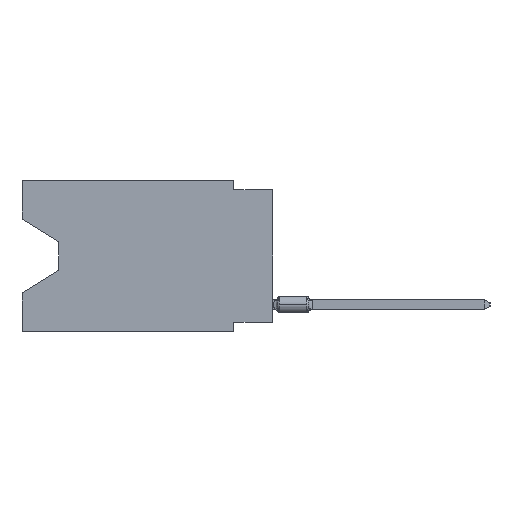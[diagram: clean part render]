
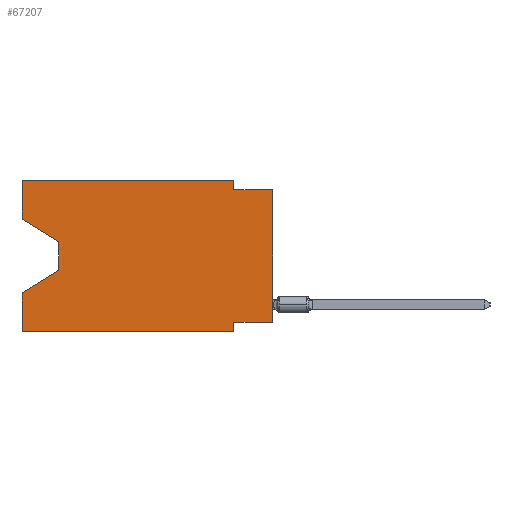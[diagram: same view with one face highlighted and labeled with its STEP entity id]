
A CAD part, left-side view. The second image highlights one B-rep face of the part: STEP entity #67207.
In plain terms, the highlighted planar face has unit normal (-1, 0, 0).
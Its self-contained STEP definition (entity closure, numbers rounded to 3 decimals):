
#865 = VECTOR ( 'NONE', #69409, 1000. ) ;
#2156 = VECTOR ( 'NONE', #59190, 1000. ) ;
#2720 = CARTESIAN_POINT ( 'NONE',  ( 0., 2.54, 0. ) ) ;
#2773 = VECTOR ( 'NONE', #17506, 1000. ) ;
#2806 = CARTESIAN_POINT ( 'NONE',  ( 0., 16.383, -7.36 ) ) ;
#4636 = DIRECTION ( 'NONE',  ( 0., 0.855, -0.519 ) ) ;
#7110 = ORIENTED_EDGE ( 'NONE', *, *, #70631, .F. ) ;
#7750 = VECTOR ( 'NONE', #42938, 1000. ) ;
#7987 = EDGE_CURVE ( 'NONE', #22921, #85334, #28754, .T. ) ;
#11176 = VECTOR ( 'NONE', #67399, 1000. ) ;
#14321 = ORIENTED_EDGE ( 'NONE', *, *, #21573, .F. ) ;
#15529 = EDGE_CURVE ( 'NONE', #75720, #67222, #23640, .T. ) ;
#15747 = CARTESIAN_POINT ( 'NONE',  ( 0., 13.97, -4.013 ) ) ;
#16799 = ORIENTED_EDGE ( 'NONE', *, *, #28957, .F. ) ;
#17506 = DIRECTION ( 'NONE',  ( 0., -1., 0. ) ) ;
#19652 = ORIENTED_EDGE ( 'NONE', *, *, #63104, .T. ) ;
#21573 = EDGE_CURVE ( 'NONE', #85607, #34274, #83770, .T. ) ;
#22626 = CARTESIAN_POINT ( 'NONE',  ( 0., 0., -9.271 ) ) ;
#22858 = VECTOR ( 'NONE', #66157, 1000. ) ;
#22921 = VERTEX_POINT ( 'NONE', #47606 ) ;
#23640 = LINE ( 'NONE', #15747, #7750 ) ;
#25227 = VERTEX_POINT ( 'NONE', #72711 ) ;
#25934 = CARTESIAN_POINT ( 'NONE',  ( 0., 2.54, -0.635 ) ) ;
#26866 = CARTESIAN_POINT ( 'NONE',  ( 0., 16.383, 0. ) ) ;
#27895 = VERTEX_POINT ( 'NONE', #2806 ) ;
#27979 = CARTESIAN_POINT ( 'NONE',  ( 0., 13.97, -4.013 ) ) ;
#28754 = LINE ( 'NONE', #55521, #61513 ) ;
#28957 = EDGE_CURVE ( 'NONE', #41726, #27895, #59170, .T. ) ;
#29472 = LINE ( 'NONE', #30329, #865 ) ;
#29495 = VERTEX_POINT ( 'NONE', #2720 ) ;
#30114 = ORIENTED_EDGE ( 'NONE', *, *, #72258, .F. ) ;
#30329 = CARTESIAN_POINT ( 'NONE',  ( 0., 16.383, -9.906 ) ) ;
#30726 = LINE ( 'NONE', #56609, #71638 ) ;
#30903 = ORIENTED_EDGE ( 'NONE', *, *, #15529, .T. ) ;
#31902 = LINE ( 'NONE', #85434, #78653 ) ;
#31994 = CARTESIAN_POINT ( 'NONE',  ( 0., 16.383, -2.546 ) ) ;
#34274 = VERTEX_POINT ( 'NONE', #86772 ) ;
#34283 = EDGE_CURVE ( 'NONE', #54685, #22921, #37753, .T. ) ;
#34741 = AXIS2_PLACEMENT_3D ( 'NONE', #49999, #68485, #36417 ) ;
#35579 = EDGE_LOOP ( 'NONE', ( #43740, #30903, #40890, #16799, #19652, #63907, #70635, #58955, #14321, #30114, #7110, #37715 ) ) ;
#35743 = LINE ( 'NONE', #40631, #11176 ) ;
#36405 = CARTESIAN_POINT ( 'NONE',  ( 0., 0., -0.635 ) ) ;
#36417 = DIRECTION ( 'NONE',  ( 0., 0., -1. ) ) ;
#37715 = ORIENTED_EDGE ( 'NONE', *, *, #39222, .F. ) ;
#37753 = LINE ( 'NONE', #71112, #22858 ) ;
#39222 = EDGE_CURVE ( 'NONE', #72754, #25227, #60225, .T. ) ;
#40631 = CARTESIAN_POINT ( 'NONE',  ( 0., 16.383, 0. ) ) ;
#40890 = ORIENTED_EDGE ( 'NONE', *, *, #60741, .T. ) ;
#41726 = VERTEX_POINT ( 'NONE', #45066 ) ;
#42938 = DIRECTION ( 'NONE',  ( 0., 0., -1. ) ) ;
#43740 = ORIENTED_EDGE ( 'NONE', *, *, #56161, .T. ) ;
#44556 = LINE ( 'NONE', #64737, #75453 ) ;
#45066 = CARTESIAN_POINT ( 'NONE',  ( 0., 16.383, -9.906 ) ) ;
#47606 = CARTESIAN_POINT ( 'NONE',  ( 0., 2.54, -9.271 ) ) ;
#49999 = CARTESIAN_POINT ( 'NONE',  ( 0., 16.383, 0. ) ) ;
#54685 = VERTEX_POINT ( 'NONE', #22626 ) ;
#55287 = FACE_OUTER_BOUND ( 'NONE', #35579, .T. ) ;
#55521 = CARTESIAN_POINT ( 'NONE',  ( 0., 2.54, -9.906 ) ) ;
#56161 = EDGE_CURVE ( 'NONE', #72754, #75720, #58296, .T. ) ;
#56609 = CARTESIAN_POINT ( 'NONE',  ( 0., 0., 0. ) ) ;
#58204 = DIRECTION ( 'NONE',  ( 0., 0., -1. ) ) ;
#58296 = LINE ( 'NONE', #31994, #2156 ) ;
#58955 = ORIENTED_EDGE ( 'NONE', *, *, #78268, .T. ) ;
#59170 = LINE ( 'NONE', #86356, #81744 ) ;
#59190 = DIRECTION ( 'NONE',  ( 0., -0.855, -0.519 ) ) ;
#59343 = DIRECTION ( 'NONE',  ( 0., 0., 1. ) ) ;
#60033 = DIRECTION ( 'NONE',  ( 0., 0., 1. ) ) ;
#60225 = LINE ( 'NONE', #26866, #74162 ) ;
#60741 = EDGE_CURVE ( 'NONE', #67222, #27895, #44556, .T. ) ;
#61513 = VECTOR ( 'NONE', #82283, 1000. ) ;
#61878 = CARTESIAN_POINT ( 'NONE',  ( 0., 13.97, -5.893 ) ) ;
#63104 = EDGE_CURVE ( 'NONE', #41726, #85334, #29472, .T. ) ;
#63907 = ORIENTED_EDGE ( 'NONE', *, *, #7987, .F. ) ;
#64737 = CARTESIAN_POINT ( 'NONE',  ( 0., 13.97, -5.893 ) ) ;
#66157 = DIRECTION ( 'NONE',  ( 0., 1., 0. ) ) ;
#67207 = ADVANCED_FACE ( 'NONE', ( #55287 ), #70206, .F. ) ;
#67222 = VERTEX_POINT ( 'NONE', #61878 ) ;
#67399 = DIRECTION ( 'NONE',  ( 0., -1., 0. ) ) ;
#68485 = DIRECTION ( 'NONE',  ( 1., 0., 0. ) ) ;
#69409 = DIRECTION ( 'NONE',  ( 0., -1., 0. ) ) ;
#70044 = CARTESIAN_POINT ( 'NONE',  ( 0., 16.383, -2.546 ) ) ;
#70206 = PLANE ( 'NONE',  #34741 ) ;
#70631 = EDGE_CURVE ( 'NONE', #25227, #29495, #35743, .T. ) ;
#70635 = ORIENTED_EDGE ( 'NONE', *, *, #34283, .F. ) ;
#71112 = CARTESIAN_POINT ( 'NONE',  ( 0., 0., -9.271 ) ) ;
#71638 = VECTOR ( 'NONE', #83367, 1000. ) ;
#72258 = EDGE_CURVE ( 'NONE', #29495, #85607, #31902, .T. ) ;
#72711 = CARTESIAN_POINT ( 'NONE',  ( 0., 16.383, 0. ) ) ;
#72754 = VERTEX_POINT ( 'NONE', #70044 ) ;
#73869 = CARTESIAN_POINT ( 'NONE',  ( 0., 2.54, -9.906 ) ) ;
#74162 = VECTOR ( 'NONE', #59343, 1000. ) ;
#75453 = VECTOR ( 'NONE', #4636, 1000. ) ;
#75720 = VERTEX_POINT ( 'NONE', #27979 ) ;
#78268 = EDGE_CURVE ( 'NONE', #54685, #34274, #30726, .T. ) ;
#78653 = VECTOR ( 'NONE', #58204, 1000. ) ;
#81744 = VECTOR ( 'NONE', #60033, 1000. ) ;
#82283 = DIRECTION ( 'NONE',  ( 0., 0., -1. ) ) ;
#83367 = DIRECTION ( 'NONE',  ( 0., 0., 1. ) ) ;
#83770 = LINE ( 'NONE', #36405, #2773 ) ;
#85334 = VERTEX_POINT ( 'NONE', #73869 ) ;
#85434 = CARTESIAN_POINT ( 'NONE',  ( 0., 2.54, 0. ) ) ;
#85607 = VERTEX_POINT ( 'NONE', #25934 ) ;
#86356 = CARTESIAN_POINT ( 'NONE',  ( 0., 16.383, 0. ) ) ;
#86772 = CARTESIAN_POINT ( 'NONE',  ( 0., 0., -0.635 ) ) ;
